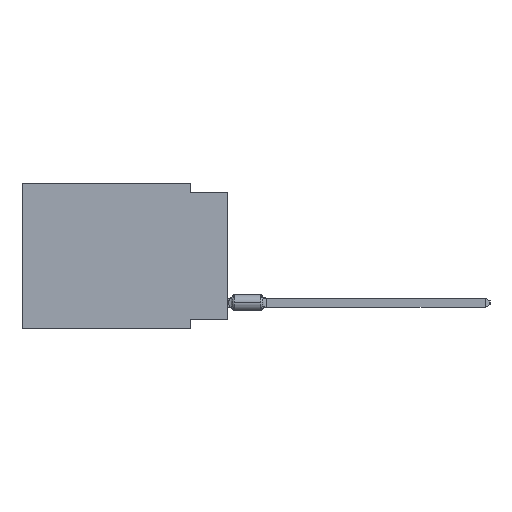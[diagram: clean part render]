
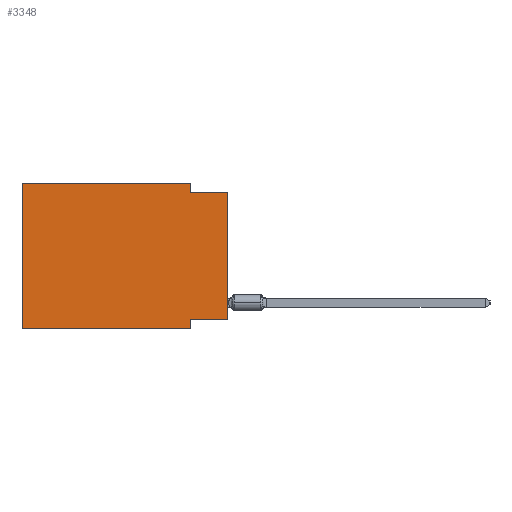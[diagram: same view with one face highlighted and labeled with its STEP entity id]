
A CAD part, left-side view. The second image highlights one B-rep face of the part: STEP entity #3348.
In plain terms, the highlighted planar face has unit normal (-1, 0, 0).
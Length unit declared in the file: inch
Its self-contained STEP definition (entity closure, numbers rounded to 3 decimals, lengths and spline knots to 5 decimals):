
#922 = CARTESIAN_POINT ( 'NONE',  ( 0., 0.1, -0.39 ) ) ;
#1024 = LINE ( 'NONE', #69909, #27573 ) ;
#1462 = ORIENTED_EDGE ( 'NONE', *, *, #8193, .F. ) ;
#2204 = VECTOR ( 'NONE', #56652, 39.37008 ) ;
#2935 = VECTOR ( 'NONE', #45631, 39.37008 ) ;
#3348 = ADVANCED_FACE ( 'NONE', ( #32690 ), #44350, .F. ) ;
#3431 = CARTESIAN_POINT ( 'NONE',  ( 0., 0.55, 0. ) ) ;
#4088 = CARTESIAN_POINT ( 'NONE',  ( 0., 0.55, 0. ) ) ;
#4187 = VERTEX_POINT ( 'NONE', #38409 ) ;
#6704 = EDGE_LOOP ( 'NONE', ( #32860, #71072, #13422, #1462, #33179, #34823, #74461, #44465 ) ) ;
#7311 = CARTESIAN_POINT ( 'NONE',  ( 0., 0.1, -0.365 ) ) ;
#7569 = VERTEX_POINT ( 'NONE', #7311 ) ;
#8193 = EDGE_CURVE ( 'NONE', #16771, #48260, #42247, .T. ) ;
#10085 = DIRECTION ( 'NONE',  ( 1., 0., 0. ) ) ;
#12645 = DIRECTION ( 'NONE',  ( 0., 0., -1. ) ) ;
#13422 = ORIENTED_EDGE ( 'NONE', *, *, #62820, .F. ) ;
#13835 = LINE ( 'NONE', #19509, #44395 ) ;
#14455 = VECTOR ( 'NONE', #69777, 39.37008 ) ;
#14953 = DIRECTION ( 'NONE',  ( 0., -1., 0. ) ) ;
#16771 = VERTEX_POINT ( 'NONE', #47532 ) ;
#17228 = LINE ( 'NONE', #46211, #71899 ) ;
#17774 = CARTESIAN_POINT ( 'NONE',  ( 0., 0., -0.025 ) ) ;
#19509 = CARTESIAN_POINT ( 'NONE',  ( 0., 0.55, -0.39 ) ) ;
#20568 = EDGE_CURVE ( 'NONE', #7569, #33246, #64842, .T. ) ;
#23505 = LINE ( 'NONE', #34032, #2204 ) ;
#23831 = CARTESIAN_POINT ( 'NONE',  ( 0., 0.1, -0.39 ) ) ;
#26392 = DIRECTION ( 'NONE',  ( 0., 0., 1. ) ) ;
#27573 = VECTOR ( 'NONE', #12645, 39.37008 ) ;
#29196 = CARTESIAN_POINT ( 'NONE',  ( 0., 0.1, 0. ) ) ;
#30770 = AXIS2_PLACEMENT_3D ( 'NONE', #4088, #10085, #67687 ) ;
#31656 = LINE ( 'NONE', #3431, #36601 ) ;
#31843 = VERTEX_POINT ( 'NONE', #44200 ) ;
#32690 = FACE_OUTER_BOUND ( 'NONE', #6704, .T. ) ;
#32860 = ORIENTED_EDGE ( 'NONE', *, *, #59697, .T. ) ;
#33179 = ORIENTED_EDGE ( 'NONE', *, *, #39773, .F. ) ;
#33246 = VERTEX_POINT ( 'NONE', #922 ) ;
#34032 = CARTESIAN_POINT ( 'NONE',  ( 0., 0., 0. ) ) ;
#34823 = ORIENTED_EDGE ( 'NONE', *, *, #62490, .T. ) ;
#35482 = DIRECTION ( 'NONE',  ( 0., 0., -1. ) ) ;
#36601 = VECTOR ( 'NONE', #26392, 39.37008 ) ;
#38409 = CARTESIAN_POINT ( 'NONE',  ( 0., 0., -0.025 ) ) ;
#39773 = EDGE_CURVE ( 'NONE', #31843, #16771, #31656, .T. ) ;
#42247 = LINE ( 'NONE', #48271, #14455 ) ;
#44004 = EDGE_CURVE ( 'NONE', #46860, #7569, #17228, .T. ) ;
#44200 = CARTESIAN_POINT ( 'NONE',  ( 0., 0.55, -0.39 ) ) ;
#44350 = PLANE ( 'NONE',  #30770 ) ;
#44395 = VECTOR ( 'NONE', #14953, 39.37008 ) ;
#44465 = ORIENTED_EDGE ( 'NONE', *, *, #44004, .F. ) ;
#45631 = DIRECTION ( 'NONE',  ( 0., -1., 0. ) ) ;
#45958 = VECTOR ( 'NONE', #35482, 39.37008 ) ;
#46211 = CARTESIAN_POINT ( 'NONE',  ( 0., 0., -0.365 ) ) ;
#46860 = VERTEX_POINT ( 'NONE', #66122 ) ;
#47532 = CARTESIAN_POINT ( 'NONE',  ( 0., 0.55, 0. ) ) ;
#47920 = CARTESIAN_POINT ( 'NONE',  ( 0., 0.1, -0.025 ) ) ;
#48260 = VERTEX_POINT ( 'NONE', #29196 ) ;
#48271 = CARTESIAN_POINT ( 'NONE',  ( 0., 0.55, 0. ) ) ;
#56652 = DIRECTION ( 'NONE',  ( 0., 0., 1. ) ) ;
#59697 = EDGE_CURVE ( 'NONE', #46860, #4187, #23505, .T. ) ;
#62189 = LINE ( 'NONE', #17774, #2935 ) ;
#62405 = DIRECTION ( 'NONE',  ( 0., 1., 0. ) ) ;
#62490 = EDGE_CURVE ( 'NONE', #31843, #33246, #13835, .T. ) ;
#62820 = EDGE_CURVE ( 'NONE', #48260, #72812, #1024, .T. ) ;
#64842 = LINE ( 'NONE', #23831, #45958 ) ;
#66122 = CARTESIAN_POINT ( 'NONE',  ( 0., 0., -0.365 ) ) ;
#67384 = EDGE_CURVE ( 'NONE', #72812, #4187, #62189, .T. ) ;
#67687 = DIRECTION ( 'NONE',  ( 0., 0., -1. ) ) ;
#69777 = DIRECTION ( 'NONE',  ( 0., -1., 0. ) ) ;
#69909 = CARTESIAN_POINT ( 'NONE',  ( 0., 0.1, 0. ) ) ;
#71072 = ORIENTED_EDGE ( 'NONE', *, *, #67384, .F. ) ;
#71899 = VECTOR ( 'NONE', #62405, 39.37008 ) ;
#72812 = VERTEX_POINT ( 'NONE', #47920 ) ;
#74461 = ORIENTED_EDGE ( 'NONE', *, *, #20568, .F. ) ;
